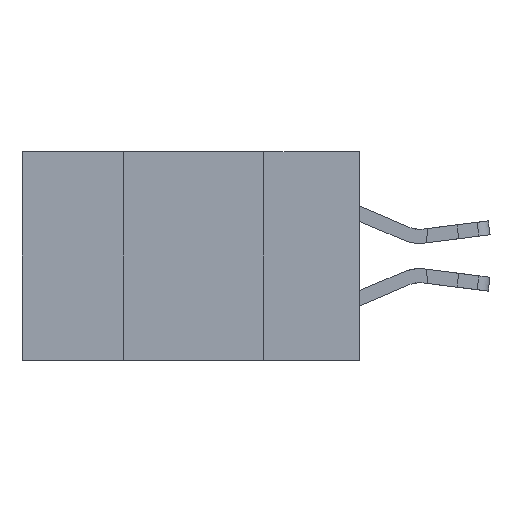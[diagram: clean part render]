
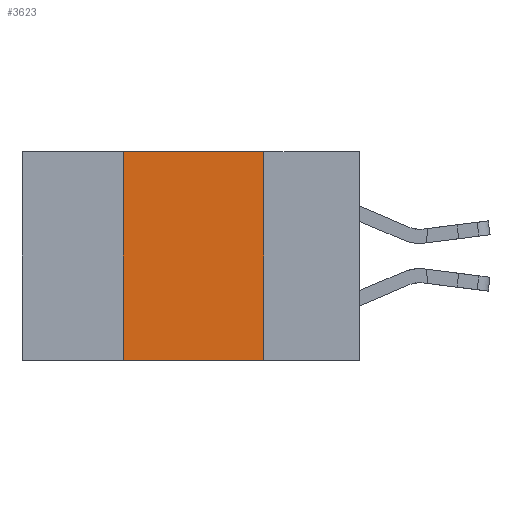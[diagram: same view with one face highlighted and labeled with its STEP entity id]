
A CAD part, left-side view. The second image highlights one B-rep face of the part: STEP entity #3623.
In plain terms, the highlighted planar face has unit normal (-1, 0, 0).
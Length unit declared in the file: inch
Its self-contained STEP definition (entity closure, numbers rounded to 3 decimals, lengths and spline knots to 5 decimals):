
#543 = EDGE_CURVE ( 'NONE', #27432, #20535, #1108, .T. ) ;
#1108 = LINE ( 'NONE', #15058, #19236 ) ;
#2889 = LINE ( 'NONE', #28422, #19204 ) ;
#3623 = ADVANCED_FACE ( 'NONE', ( #8409 ), #11222, .F. ) ;
#5145 = DIRECTION ( 'NONE',  ( 0., -1., 0. ) ) ;
#5263 = VERTEX_POINT ( 'NONE', #31721 ) ;
#6427 = ORIENTED_EDGE ( 'NONE', *, *, #543, .T. ) ;
#6819 = ORIENTED_EDGE ( 'NONE', *, *, #22874, .F. ) ;
#8409 = FACE_OUTER_BOUND ( 'NONE', #9025, .T. ) ;
#9025 = EDGE_LOOP ( 'NONE', ( #15351, #6819, #24867, #6427 ) ) ;
#11222 = PLANE ( 'NONE',  #32016 ) ;
#11309 = CARTESIAN_POINT ( 'NONE',  ( 0., 0.17, 0. ) ) ;
#11878 = VERTEX_POINT ( 'NONE', #11309 ) ;
#12727 = DIRECTION ( 'NONE',  ( 0., -1., 0. ) ) ;
#14382 = VECTOR ( 'NONE', #20737, 39.37008 ) ;
#15058 = CARTESIAN_POINT ( 'NONE',  ( 0., 0.6, -0.37 ) ) ;
#15351 = ORIENTED_EDGE ( 'NONE', *, *, #29087, .F. ) ;
#15530 = LINE ( 'NONE', #25569, #15700 ) ;
#15700 = VECTOR ( 'NONE', #12727, 39.37008 ) ;
#16659 = CARTESIAN_POINT ( 'NONE',  ( 0., 0.6, 0. ) ) ;
#18242 = EDGE_CURVE ( 'NONE', #27432, #5263, #2889, .T. ) ;
#18809 = DIRECTION ( 'NONE',  ( 1., 0., 0. ) ) ;
#19204 = VECTOR ( 'NONE', #20554, 39.37008 ) ;
#19236 = VECTOR ( 'NONE', #5145, 39.37008 ) ;
#20535 = VERTEX_POINT ( 'NONE', #27867 ) ;
#20554 = DIRECTION ( 'NONE',  ( 0., 0., 1. ) ) ;
#20737 = DIRECTION ( 'NONE',  ( 0., 0., -1. ) ) ;
#22874 = EDGE_CURVE ( 'NONE', #5263, #11878, #15530, .T. ) ;
#23409 = DIRECTION ( 'NONE',  ( 0., 0., -1. ) ) ;
#24867 = ORIENTED_EDGE ( 'NONE', *, *, #18242, .F. ) ;
#25218 = CARTESIAN_POINT ( 'NONE',  ( 0., 0.42, -0.37 ) ) ;
#25569 = CARTESIAN_POINT ( 'NONE',  ( 0., 0.6, 0. ) ) ;
#25818 = CARTESIAN_POINT ( 'NONE',  ( 0., 0.17, 0. ) ) ;
#27432 = VERTEX_POINT ( 'NONE', #25218 ) ;
#27867 = CARTESIAN_POINT ( 'NONE',  ( 0., 0.17, -0.37 ) ) ;
#28422 = CARTESIAN_POINT ( 'NONE',  ( 0., 0.42, 0. ) ) ;
#29087 = EDGE_CURVE ( 'NONE', #11878, #20535, #30269, .T. ) ;
#30269 = LINE ( 'NONE', #25818, #14382 ) ;
#31721 = CARTESIAN_POINT ( 'NONE',  ( 0., 0.42, 0. ) ) ;
#32016 = AXIS2_PLACEMENT_3D ( 'NONE', #16659, #18809, #23409 ) ;
